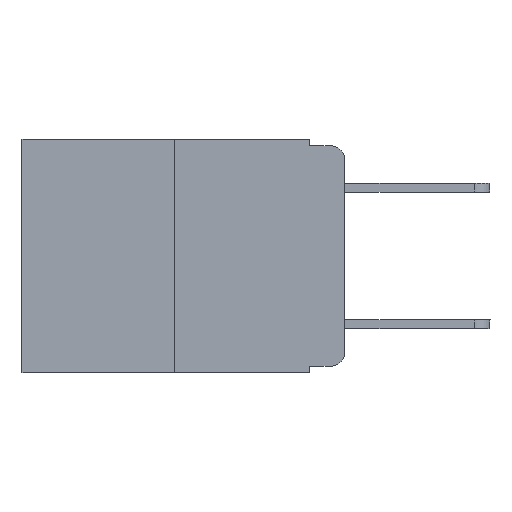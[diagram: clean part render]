
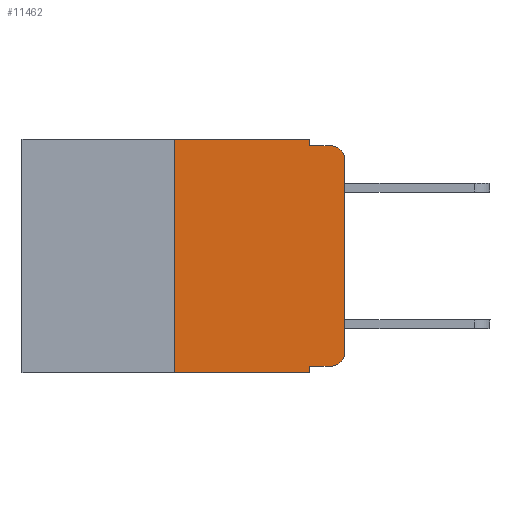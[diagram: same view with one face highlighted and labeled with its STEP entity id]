
A CAD part, left-side view. The second image highlights one B-rep face of the part: STEP entity #11462.
In plain terms, the highlighted planar face has unit normal (-1, 0, 0).
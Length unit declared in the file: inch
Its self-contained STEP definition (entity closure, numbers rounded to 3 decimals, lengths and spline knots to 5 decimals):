
#237 = VERTEX_POINT ( 'NONE', #7211 ) ;
#923 = EDGE_CURVE ( 'NONE', #1381, #237, #12223, .T. ) ;
#993 = CARTESIAN_POINT ( 'NONE',  ( 0., 0.051, -0.333 ) ) ;
#999 = VECTOR ( 'NONE', #8053, 39.37008 ) ;
#1077 = CARTESIAN_POINT ( 'NONE',  ( 0., 0.02, -0.01 ) ) ;
#1141 = DIRECTION ( 'NONE',  ( 0., 0., 1. ) ) ;
#1223 = LINE ( 'NONE', #3883, #999 ) ;
#1381 = VERTEX_POINT ( 'NONE', #11223 ) ;
#1852 = VERTEX_POINT ( 'NONE', #18132 ) ;
#1885 = VECTOR ( 'NONE', #16101, 39.37008 ) ;
#1914 = CARTESIAN_POINT ( 'NONE',  ( 0., 0.473, 0. ) ) ;
#1992 = EDGE_CURVE ( 'NONE', #1852, #4862, #1223, .T. ) ;
#1993 = EDGE_CURVE ( 'NONE', #10302, #13322, #16383, .T. ) ;
#1998 = LINE ( 'NONE', #4624, #6797 ) ;
#2198 = CARTESIAN_POINT ( 'NONE',  ( 0., 0.25, 0. ) ) ;
#2232 = ORIENTED_EDGE ( 'NONE', *, *, #7744, .T. ) ;
#3163 = PLANE ( 'NONE',  #14662 ) ;
#3434 = VERTEX_POINT ( 'NONE', #2198 ) ;
#3847 = CARTESIAN_POINT ( 'NONE',  ( 0., 0.25, 0. ) ) ;
#3883 = CARTESIAN_POINT ( 'NONE',  ( 0., 0.051, -0.01 ) ) ;
#4624 = CARTESIAN_POINT ( 'NONE',  ( 0., 0.051, 0. ) ) ;
#4733 = DIRECTION ( 'NONE',  ( 0., 0., -1. ) ) ;
#4862 = VERTEX_POINT ( 'NONE', #1077 ) ;
#4927 = EDGE_CURVE ( 'NONE', #9062, #3434, #14753, .T. ) ;
#5264 = DIRECTION ( 'NONE',  ( 0., 0., -1. ) ) ;
#5298 = DIRECTION ( 'NONE',  ( 0., 0., 1. ) ) ;
#5711 = CARTESIAN_POINT ( 'NONE',  ( 0., 0.051, -0.343 ) ) ;
#5807 = ORIENTED_EDGE ( 'NONE', *, *, #923, .T. ) ;
#5845 = VECTOR ( 'NONE', #5298, 39.37008 ) ;
#6210 = EDGE_LOOP ( 'NONE', ( #2232, #15584, #6332, #7230, #15435, #6519, #11410, #17023, #9503, #5807 ) ) ;
#6332 = ORIENTED_EDGE ( 'NONE', *, *, #1992, .F. ) ;
#6511 = AXIS2_PLACEMENT_3D ( 'NONE', #11860, #14677, #13428 ) ;
#6519 = ORIENTED_EDGE ( 'NONE', *, *, #4927, .F. ) ;
#6679 = EDGE_CURVE ( 'NONE', #9062, #13322, #8282, .T. ) ;
#6797 = VECTOR ( 'NONE', #4733, 39.37008 ) ;
#6831 = DIRECTION ( 'NONE',  ( 0., -1., 0. ) ) ;
#7050 = VECTOR ( 'NONE', #8058, 39.37008 ) ;
#7211 = CARTESIAN_POINT ( 'NONE',  ( 0., 0., -0.313 ) ) ;
#7230 = ORIENTED_EDGE ( 'NONE', *, *, #16765, .F. ) ;
#7386 = DIRECTION ( 'NONE',  ( -1., 0., 0. ) ) ;
#7744 = EDGE_CURVE ( 'NONE', #237, #11876, #10426, .T. ) ;
#7816 = FACE_OUTER_BOUND ( 'NONE', #6210, .T. ) ;
#8053 = DIRECTION ( 'NONE',  ( 0., -1., 0. ) ) ;
#8058 = DIRECTION ( 'NONE',  ( 0., -1., 0. ) ) ;
#8230 = CARTESIAN_POINT ( 'NONE',  ( 0., 0.051, 0. ) ) ;
#8282 = LINE ( 'NONE', #17389, #12930 ) ;
#8411 = CARTESIAN_POINT ( 'NONE',  ( 0., 0.051, -0.333 ) ) ;
#8713 = DIRECTION ( 'NONE',  ( 0., 0., -1. ) ) ;
#9062 = VERTEX_POINT ( 'NONE', #14809 ) ;
#9491 = CIRCLE ( 'NONE', #13223, 0.02 ) ;
#9503 = ORIENTED_EDGE ( 'NONE', *, *, #15726, .T. ) ;
#10185 = DIRECTION ( 'NONE',  ( 0., 0., -1. ) ) ;
#10302 = VERTEX_POINT ( 'NONE', #8411 ) ;
#10426 = LINE ( 'NONE', #12396, #5845 ) ;
#10487 = EDGE_CURVE ( 'NONE', #11876, #4862, #9491, .T. ) ;
#10686 = VERTEX_POINT ( 'NONE', #8230 ) ;
#10778 = LINE ( 'NONE', #993, #7050 ) ;
#10966 = VECTOR ( 'NONE', #1141, 39.37008 ) ;
#11223 = CARTESIAN_POINT ( 'NONE',  ( 0., 0.02, -0.333 ) ) ;
#11410 = ORIENTED_EDGE ( 'NONE', *, *, #6679, .T. ) ;
#11462 = ADVANCED_FACE ( 'NONE', ( #7816 ), #3163, .F. ) ;
#11724 = LINE ( 'NONE', #1914, #1885 ) ;
#11860 = CARTESIAN_POINT ( 'NONE',  ( 0., 0.02, -0.313 ) ) ;
#11876 = VERTEX_POINT ( 'NONE', #13519 ) ;
#12223 = CIRCLE ( 'NONE', #6511, 0.02 ) ;
#12396 = CARTESIAN_POINT ( 'NONE',  ( 0., 0., 0. ) ) ;
#12804 = CARTESIAN_POINT ( 'NONE',  ( 0., 0.473, 0. ) ) ;
#12922 = EDGE_CURVE ( 'NONE', #3434, #10686, #11724, .T. ) ;
#12930 = VECTOR ( 'NONE', #6831, 39.37008 ) ;
#13223 = AXIS2_PLACEMENT_3D ( 'NONE', #15845, #7386, #10185 ) ;
#13303 = VECTOR ( 'NONE', #5264, 39.37008 ) ;
#13322 = VERTEX_POINT ( 'NONE', #5711 ) ;
#13428 = DIRECTION ( 'NONE',  ( 0., 0., -1. ) ) ;
#13519 = CARTESIAN_POINT ( 'NONE',  ( 0., 0., -0.03 ) ) ;
#13688 = CARTESIAN_POINT ( 'NONE',  ( 0., 0.051, 0. ) ) ;
#14384 = DIRECTION ( 'NONE',  ( 1., 0., 0. ) ) ;
#14662 = AXIS2_PLACEMENT_3D ( 'NONE', #12804, #14384, #8713 ) ;
#14677 = DIRECTION ( 'NONE',  ( -1., 0., 0. ) ) ;
#14753 = LINE ( 'NONE', #3847, #10966 ) ;
#14809 = CARTESIAN_POINT ( 'NONE',  ( 0., 0.25, -0.343 ) ) ;
#15435 = ORIENTED_EDGE ( 'NONE', *, *, #12922, .F. ) ;
#15584 = ORIENTED_EDGE ( 'NONE', *, *, #10487, .T. ) ;
#15726 = EDGE_CURVE ( 'NONE', #10302, #1381, #10778, .T. ) ;
#15845 = CARTESIAN_POINT ( 'NONE',  ( 0., 0.02, -0.03 ) ) ;
#16101 = DIRECTION ( 'NONE',  ( 0., -1., 0. ) ) ;
#16383 = LINE ( 'NONE', #13688, #13303 ) ;
#16765 = EDGE_CURVE ( 'NONE', #10686, #1852, #1998, .T. ) ;
#17023 = ORIENTED_EDGE ( 'NONE', *, *, #1993, .F. ) ;
#17389 = CARTESIAN_POINT ( 'NONE',  ( 0., 0.473, -0.343 ) ) ;
#18132 = CARTESIAN_POINT ( 'NONE',  ( 0., 0.051, -0.01 ) ) ;
